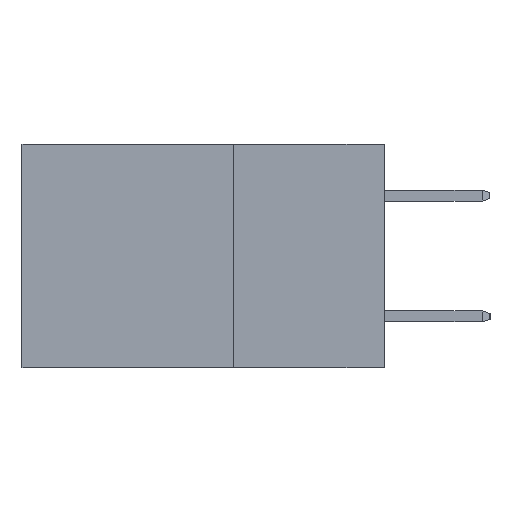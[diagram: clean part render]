
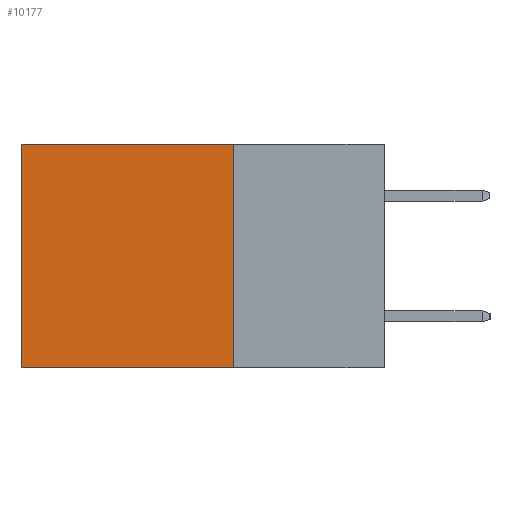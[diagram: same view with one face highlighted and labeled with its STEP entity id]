
A CAD part, left-side view. The second image highlights one B-rep face of the part: STEP entity #10177.
In plain terms, the highlighted planar face has unit normal (-1, 0, 0).
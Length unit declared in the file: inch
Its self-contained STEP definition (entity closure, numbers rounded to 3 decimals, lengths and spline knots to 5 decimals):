
#393 = DIRECTION ( 'NONE',  ( 0., 1., 0. ) ) ;
#439 = LINE ( 'NONE', #2012, #8720 ) ;
#1187 = VECTOR ( 'NONE', #6405, 39.37008 ) ;
#1448 = DIRECTION ( 'NONE',  ( 0., 0., -1. ) ) ;
#1664 = VERTEX_POINT ( 'NONE', #7516 ) ;
#1781 = VECTOR ( 'NONE', #9037, 39.37008 ) ;
#1934 = CARTESIAN_POINT ( 'NONE',  ( 0.2615, 0.25, 0. ) ) ;
#2007 = EDGE_CURVE ( 'NONE', #5596, #7786, #5536, .T. ) ;
#2012 = CARTESIAN_POINT ( 'NONE',  ( 0.2615, 0.25, -0.37 ) ) ;
#2045 = EDGE_LOOP ( 'NONE', ( #4783, #4976, #5027, #5491 ) ) ;
#2113 = PLANE ( 'NONE',  #9770 ) ;
#2854 = EDGE_CURVE ( 'NONE', #5596, #1664, #10097, .T. ) ;
#2940 = DIRECTION ( 'NONE',  ( 1., 0., 0. ) ) ;
#3373 = CARTESIAN_POINT ( 'NONE',  ( 0.2615, 0.6, 0. ) ) ;
#4201 = LINE ( 'NONE', #6703, #1781 ) ;
#4783 = ORIENTED_EDGE ( 'NONE', *, *, #8321, .T. ) ;
#4976 = ORIENTED_EDGE ( 'NONE', *, *, #5500, .F. ) ;
#5027 = ORIENTED_EDGE ( 'NONE', *, *, #2854, .F. ) ;
#5250 = VERTEX_POINT ( 'NONE', #9688 ) ;
#5491 = ORIENTED_EDGE ( 'NONE', *, *, #2007, .T. ) ;
#5500 = EDGE_CURVE ( 'NONE', #1664, #5250, #439, .T. ) ;
#5536 = LINE ( 'NONE', #1934, #1187 ) ;
#5596 = VERTEX_POINT ( 'NONE', #6960 ) ;
#6405 = DIRECTION ( 'NONE',  ( 0., 1., 0. ) ) ;
#6646 = CARTESIAN_POINT ( 'NONE',  ( 0.2615, 0.25, -0.37 ) ) ;
#6703 = CARTESIAN_POINT ( 'NONE',  ( 0.2615, 0.6, -0.37 ) ) ;
#6960 = CARTESIAN_POINT ( 'NONE',  ( 0.2615, 0.25, 0. ) ) ;
#7516 = CARTESIAN_POINT ( 'NONE',  ( 0.2615, 0.25, -0.37 ) ) ;
#7652 = FACE_OUTER_BOUND ( 'NONE', #2045, .T. ) ;
#7786 = VERTEX_POINT ( 'NONE', #3373 ) ;
#8076 = VECTOR ( 'NONE', #1448, 39.37008 ) ;
#8321 = EDGE_CURVE ( 'NONE', #7786, #5250, #4201, .T. ) ;
#8499 = DIRECTION ( 'NONE',  ( 0., 0., -1. ) ) ;
#8720 = VECTOR ( 'NONE', #393, 39.37008 ) ;
#9037 = DIRECTION ( 'NONE',  ( 0., 0., -1. ) ) ;
#9244 = CARTESIAN_POINT ( 'NONE',  ( 0.2615, 0.25, -0.37 ) ) ;
#9688 = CARTESIAN_POINT ( 'NONE',  ( 0.2615, 0.6, -0.37 ) ) ;
#9770 = AXIS2_PLACEMENT_3D ( 'NONE', #9244, #2940, #8499 ) ;
#10097 = LINE ( 'NONE', #6646, #8076 ) ;
#10177 = ADVANCED_FACE ( 'NONE', ( #7652 ), #2113, .F. ) ;
